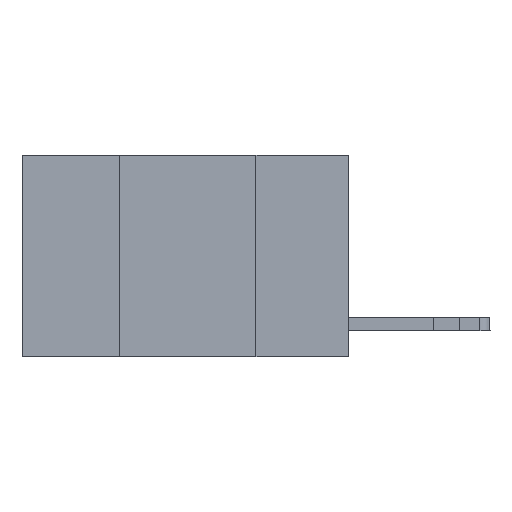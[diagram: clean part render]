
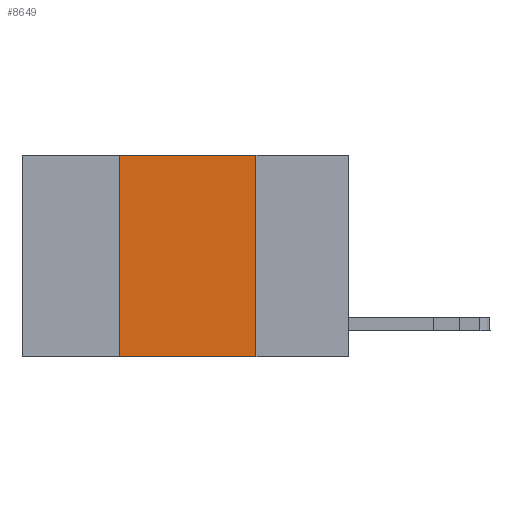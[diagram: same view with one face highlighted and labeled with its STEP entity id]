
A CAD part, left-side view. The second image highlights one B-rep face of the part: STEP entity #8649.
In plain terms, the highlighted planar face has unit normal (-1, 0, 0).
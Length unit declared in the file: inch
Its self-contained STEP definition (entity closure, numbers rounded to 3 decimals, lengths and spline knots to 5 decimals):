
#35 = DIRECTION ( 'NONE',  ( 0., 0., 1. ) ) ;
#79 = CARTESIAN_POINT ( 'NONE',  ( 0., 0.6, -0.37 ) ) ;
#1065 = PLANE ( 'NONE',  #4215 ) ;
#1165 = LINE ( 'NONE', #12805, #10146 ) ;
#1201 = VECTOR ( 'NONE', #11256, 39.37008 ) ;
#1279 = CARTESIAN_POINT ( 'NONE',  ( 0., 0.17, -0.37 ) ) ;
#1666 = CARTESIAN_POINT ( 'NONE',  ( 0., 0.17, 0. ) ) ;
#2863 = VECTOR ( 'NONE', #9859, 39.37008 ) ;
#3345 = VECTOR ( 'NONE', #35, 39.37008 ) ;
#3891 = ORIENTED_EDGE ( 'NONE', *, *, #6364, .F. ) ;
#3899 = CARTESIAN_POINT ( 'NONE',  ( 0., 0.42, -0.37 ) ) ;
#4077 = FACE_OUTER_BOUND ( 'NONE', #12515, .T. ) ;
#4215 = AXIS2_PLACEMENT_3D ( 'NONE', #5152, #12307, #7283 ) ;
#4698 = VERTEX_POINT ( 'NONE', #5848 ) ;
#5152 = CARTESIAN_POINT ( 'NONE',  ( 0., 0.6, 0. ) ) ;
#5231 = VERTEX_POINT ( 'NONE', #3899 ) ;
#5848 = CARTESIAN_POINT ( 'NONE',  ( 0., 0.42, 0. ) ) ;
#6105 = LINE ( 'NONE', #79, #1201 ) ;
#6364 = EDGE_CURVE ( 'NONE', #4698, #7138, #1165, .T. ) ;
#6393 = EDGE_CURVE ( 'NONE', #7138, #8235, #10853, .T. ) ;
#7138 = VERTEX_POINT ( 'NONE', #1666 ) ;
#7283 = DIRECTION ( 'NONE',  ( 0., 0., -1. ) ) ;
#7475 = ORIENTED_EDGE ( 'NONE', *, *, #6393, .F. ) ;
#7837 = EDGE_CURVE ( 'NONE', #5231, #4698, #11486, .T. ) ;
#8232 = EDGE_CURVE ( 'NONE', #5231, #8235, #6105, .T. ) ;
#8235 = VERTEX_POINT ( 'NONE', #1279 ) ;
#8649 = ADVANCED_FACE ( 'NONE', ( #4077 ), #1065, .F. ) ;
#9096 = ORIENTED_EDGE ( 'NONE', *, *, #7837, .F. ) ;
#9859 = DIRECTION ( 'NONE',  ( 0., 0., -1. ) ) ;
#10146 = VECTOR ( 'NONE', #10469, 39.37008 ) ;
#10466 = CARTESIAN_POINT ( 'NONE',  ( 0., 0.42, 0. ) ) ;
#10469 = DIRECTION ( 'NONE',  ( 0., -1., 0. ) ) ;
#10853 = LINE ( 'NONE', #13078, #2863 ) ;
#11256 = DIRECTION ( 'NONE',  ( 0., -1., 0. ) ) ;
#11486 = LINE ( 'NONE', #10466, #3345 ) ;
#12307 = DIRECTION ( 'NONE',  ( 1., 0., 0. ) ) ;
#12322 = ORIENTED_EDGE ( 'NONE', *, *, #8232, .T. ) ;
#12515 = EDGE_LOOP ( 'NONE', ( #7475, #3891, #9096, #12322 ) ) ;
#12805 = CARTESIAN_POINT ( 'NONE',  ( 0., 0.6, 0. ) ) ;
#13078 = CARTESIAN_POINT ( 'NONE',  ( 0., 0.17, 0. ) ) ;
